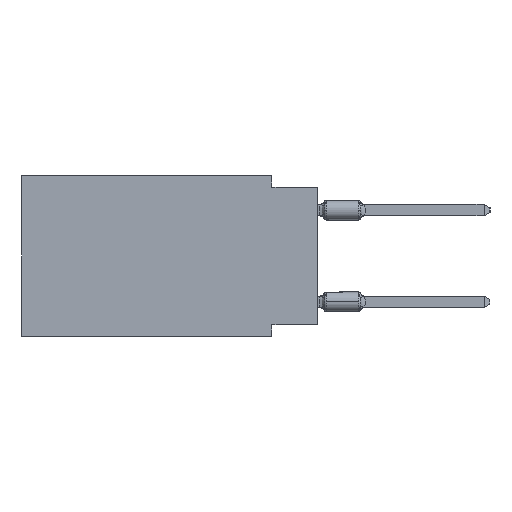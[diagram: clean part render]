
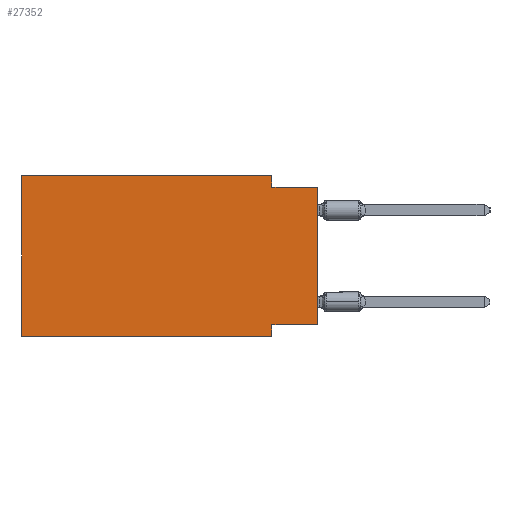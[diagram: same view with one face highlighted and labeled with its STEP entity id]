
A CAD part, left-side view. The second image highlights one B-rep face of the part: STEP entity #27352.
In plain terms, the highlighted planar face has unit normal (-1, 0, 0).
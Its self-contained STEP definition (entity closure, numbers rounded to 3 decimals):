
#1208 = EDGE_CURVE ( 'NONE', #17818, #16371, #28395, .T. ) ;
#1579 = CARTESIAN_POINT ( 'NONE',  ( 0., 2.54, 0. ) ) ;
#1989 = CARTESIAN_POINT ( 'NONE',  ( 0., 0., -8.255 ) ) ;
#2042 = LINE ( 'NONE', #12272, #21879 ) ;
#2128 = VERTEX_POINT ( 'NONE', #18687 ) ;
#2129 = VERTEX_POINT ( 'NONE', #4030 ) ;
#2327 = EDGE_CURVE ( 'NONE', #2129, #23025, #2042, .T. ) ;
#2774 = LINE ( 'NONE', #12849, #4390 ) ;
#3754 = DIRECTION ( 'NONE',  ( 0., -1., 0. ) ) ;
#3802 = CARTESIAN_POINT ( 'NONE',  ( 0., 2.54, -0.635 ) ) ;
#4030 = CARTESIAN_POINT ( 'NONE',  ( 0., 16.383, -8.89 ) ) ;
#4390 = VECTOR ( 'NONE', #8706, 1000. ) ;
#4480 = VERTEX_POINT ( 'NONE', #25376 ) ;
#5396 = CARTESIAN_POINT ( 'NONE',  ( 0., 2.54, -8.89 ) ) ;
#5815 = VECTOR ( 'NONE', #28628, 1000. ) ;
#6377 = EDGE_CURVE ( 'NONE', #2129, #2128, #27157, .T. ) ;
#6593 = DIRECTION ( 'NONE',  ( 0., -1., 0. ) ) ;
#7748 = EDGE_CURVE ( 'NONE', #16371, #23025, #2774, .T. ) ;
#7823 = EDGE_CURVE ( 'NONE', #27893, #4480, #30781, .T. ) ;
#8226 = CARTESIAN_POINT ( 'NONE',  ( 0., 0., -0.635 ) ) ;
#8522 = CARTESIAN_POINT ( 'NONE',  ( 0., 0., 0. ) ) ;
#8706 = DIRECTION ( 'NONE',  ( 0., 0., -1. ) ) ;
#9091 = CARTESIAN_POINT ( 'NONE',  ( 0., 16.383, 0. ) ) ;
#9250 = CARTESIAN_POINT ( 'NONE',  ( 0., 16.383, 0. ) ) ;
#10149 = VECTOR ( 'NONE', #3754, 1000. ) ;
#10296 = ORIENTED_EDGE ( 'NONE', *, *, #7748, .F. ) ;
#11547 = FACE_OUTER_BOUND ( 'NONE', #26712, .T. ) ;
#11643 = DIRECTION ( 'NONE',  ( 0., 0., -1. ) ) ;
#12110 = DIRECTION ( 'NONE',  ( 0., -1., 0. ) ) ;
#12272 = CARTESIAN_POINT ( 'NONE',  ( 0., 16.383, -8.89 ) ) ;
#12563 = ORIENTED_EDGE ( 'NONE', *, *, #7823, .F. ) ;
#12579 = CARTESIAN_POINT ( 'NONE',  ( 0., 2.54, 0. ) ) ;
#12813 = ORIENTED_EDGE ( 'NONE', *, *, #6377, .F. ) ;
#12849 = CARTESIAN_POINT ( 'NONE',  ( 0., 2.54, -8.89 ) ) ;
#13421 = EDGE_CURVE ( 'NONE', #32272, #27893, #29109, .T. ) ;
#14988 = ORIENTED_EDGE ( 'NONE', *, *, #1208, .F. ) ;
#15550 = DIRECTION ( 'NONE',  ( 0., 1., 0. ) ) ;
#16371 = VERTEX_POINT ( 'NONE', #29143 ) ;
#17466 = AXIS2_PLACEMENT_3D ( 'NONE', #9091, #19124, #29189 ) ;
#17818 = VERTEX_POINT ( 'NONE', #1989 ) ;
#18687 = CARTESIAN_POINT ( 'NONE',  ( 0., 16.383, 0. ) ) ;
#19124 = DIRECTION ( 'NONE',  ( 1., 0., 0. ) ) ;
#21204 = LINE ( 'NONE', #8522, #5815 ) ;
#21350 = ORIENTED_EDGE ( 'NONE', *, *, #28983, .T. ) ;
#21613 = PLANE ( 'NONE',  #17466 ) ;
#21869 = CARTESIAN_POINT ( 'NONE',  ( 0., 16.383, 0. ) ) ;
#21879 = VECTOR ( 'NONE', #12110, 1000. ) ;
#22003 = VECTOR ( 'NONE', #11643, 1000. ) ;
#22403 = ORIENTED_EDGE ( 'NONE', *, *, #13421, .F. ) ;
#22645 = CARTESIAN_POINT ( 'NONE',  ( 0., 0., -8.255 ) ) ;
#23025 = VERTEX_POINT ( 'NONE', #5396 ) ;
#24849 = VECTOR ( 'NONE', #32393, 1000. ) ;
#25376 = CARTESIAN_POINT ( 'NONE',  ( 0., 0., -0.635 ) ) ;
#26550 = VECTOR ( 'NONE', #15550, 1000. ) ;
#26712 = EDGE_LOOP ( 'NONE', ( #21350, #12563, #22403, #30388, #12813, #31305, #10296, #14988 ) ) ;
#27157 = LINE ( 'NONE', #21869, #24849 ) ;
#27186 = EDGE_CURVE ( 'NONE', #2128, #32272, #31800, .T. ) ;
#27352 = ADVANCED_FACE ( 'NONE', ( #11547 ), #21613, .F. ) ;
#27893 = VERTEX_POINT ( 'NONE', #3802 ) ;
#27991 = VECTOR ( 'NONE', #6593, 1000. ) ;
#28395 = LINE ( 'NONE', #22645, #26550 ) ;
#28628 = DIRECTION ( 'NONE',  ( 0., 0., 1. ) ) ;
#28983 = EDGE_CURVE ( 'NONE', #17818, #4480, #21204, .T. ) ;
#29109 = LINE ( 'NONE', #1579, #22003 ) ;
#29143 = CARTESIAN_POINT ( 'NONE',  ( 0., 2.54, -8.255 ) ) ;
#29189 = DIRECTION ( 'NONE',  ( 0., 0., -1. ) ) ;
#30388 = ORIENTED_EDGE ( 'NONE', *, *, #27186, .F. ) ;
#30781 = LINE ( 'NONE', #8226, #10149 ) ;
#31305 = ORIENTED_EDGE ( 'NONE', *, *, #2327, .T. ) ;
#31800 = LINE ( 'NONE', #9250, #27991 ) ;
#32272 = VERTEX_POINT ( 'NONE', #12579 ) ;
#32393 = DIRECTION ( 'NONE',  ( 0., 0., 1. ) ) ;
